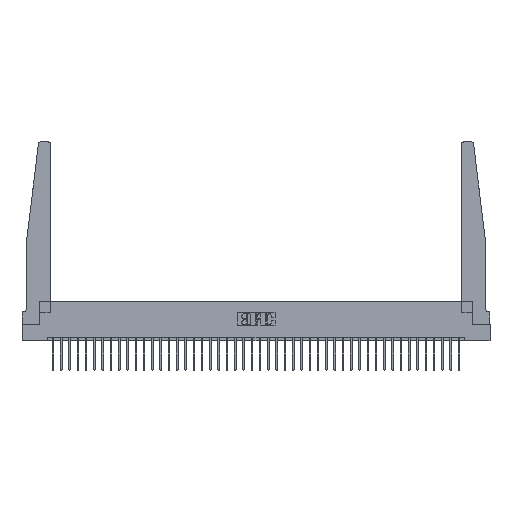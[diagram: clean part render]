
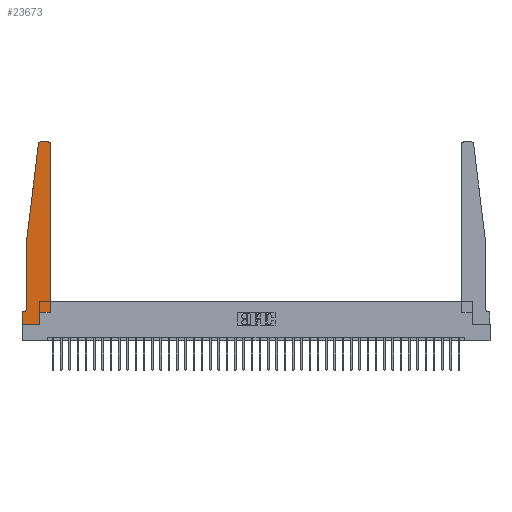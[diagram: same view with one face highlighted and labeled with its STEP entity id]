
A CAD part, top view. The second image highlights one B-rep face of the part: STEP entity #23673.
In plain terms, the highlighted planar face has unit normal (0, 0, 1).
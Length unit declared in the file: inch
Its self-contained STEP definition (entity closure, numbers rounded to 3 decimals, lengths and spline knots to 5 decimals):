
#261 = EDGE_LOOP ( 'NONE', ( #20684, #26477, #16631, #6091, #30524, #27600, #25866, #5834, #3191, #8412, #11395, #14892 ) ) ;
#293 = CARTESIAN_POINT ( 'NONE',  ( 0., 0.1875, 0.37 ) ) ;
#601 = DIRECTION ( 'NONE',  ( 1., 0., 0. ) ) ;
#1388 = CARTESIAN_POINT ( 'NONE',  ( 0.065, 1.25, 0.37 ) ) ;
#1584 = AXIS2_PLACEMENT_3D ( 'NONE', #11015, #36303, #19502 ) ;
#1932 = CARTESIAN_POINT ( 'NONE',  ( 0.395, 2.75, 0.37 ) ) ;
#2419 = EDGE_CURVE ( 'NONE', #19252, #33587, #9797, .T. ) ;
#3022 = VERTEX_POINT ( 'NONE', #9951 ) ;
#3074 = VERTEX_POINT ( 'NONE', #13169 ) ;
#3191 = ORIENTED_EDGE ( 'NONE', *, *, #34899, .T. ) ;
#4273 = EDGE_CURVE ( 'NONE', #20313, #17074, #19392, .T. ) ;
#4833 = DIRECTION ( 'NONE',  ( -1., 0., 0. ) ) ;
#5473 = CARTESIAN_POINT ( 'NONE',  ( 0.015, 0.1875, 0.37 ) ) ;
#5834 = ORIENTED_EDGE ( 'NONE', *, *, #20996, .T. ) ;
#6091 = ORIENTED_EDGE ( 'NONE', *, *, #18417, .T. ) ;
#6622 = VECTOR ( 'NONE', #32707, 39.37008 ) ;
#6654 = DIRECTION ( 'NONE',  ( 0., 1., 0. ) ) ;
#6758 = EDGE_CURVE ( 'NONE', #3022, #12682, #29801, .T. ) ;
#8298 = AXIS2_PLACEMENT_3D ( 'NONE', #293, #34190, #30541 ) ;
#8412 = ORIENTED_EDGE ( 'NONE', *, *, #4273, .T. ) ;
#8420 = LINE ( 'NONE', #16479, #15022 ) ;
#8634 = VERTEX_POINT ( 'NONE', #17667 ) ;
#8946 = EDGE_CURVE ( 'NONE', #20688, #19252, #32257, .T. ) ;
#9797 = CIRCLE ( 'NONE', #1584, 0.03 ) ;
#9951 = CARTESIAN_POINT ( 'NONE',  ( 0., 0.1875, 0.37 ) ) ;
#11015 = CARTESIAN_POINT ( 'NONE',  ( 0.27653, 2.72, 0.37 ) ) ;
#11395 = ORIENTED_EDGE ( 'NONE', *, *, #22938, .T. ) ;
#12236 = CARTESIAN_POINT ( 'NONE',  ( 0.2605, 0.18, 0.37 ) ) ;
#12353 = CARTESIAN_POINT ( 'NONE',  ( 0.27653, 2.75, 0.37 ) ) ;
#12682 = VERTEX_POINT ( 'NONE', #31662 ) ;
#13169 = CARTESIAN_POINT ( 'NONE',  ( 0.065, 1.25, 0.37 ) ) ;
#14366 = CARTESIAN_POINT ( 'NONE',  ( 0., 0., 0.37 ) ) ;
#14892 = ORIENTED_EDGE ( 'NONE', *, *, #35914, .T. ) ;
#15022 = VECTOR ( 'NONE', #22099, 39.37008 ) ;
#15377 = CARTESIAN_POINT ( 'NONE',  ( 0.425, 0.18, 0.37 ) ) ;
#15450 = EDGE_CURVE ( 'NONE', #31103, #17397, #20137, .T. ) ;
#15688 = CARTESIAN_POINT ( 'NONE',  ( 0.065, 0.1875, 0.37 ) ) ;
#16479 = CARTESIAN_POINT ( 'NONE',  ( 0.425, 0.18, 0.37 ) ) ;
#16631 = ORIENTED_EDGE ( 'NONE', *, *, #23407, .T. ) ;
#17039 = CIRCLE ( 'NONE', #25941, 0.03 ) ;
#17074 = VERTEX_POINT ( 'NONE', #15377 ) ;
#17328 = CARTESIAN_POINT ( 'NONE',  ( 0.395, 2.72, 0.37 ) ) ;
#17397 = VERTEX_POINT ( 'NONE', #5473 ) ;
#17667 = CARTESIAN_POINT ( 'NONE',  ( 0.2605, 0., 0.37 ) ) ;
#18417 = EDGE_CURVE ( 'NONE', #3074, #31103, #34608, .T. ) ;
#18793 = CARTESIAN_POINT ( 'NONE',  ( 0.425, 2.72, 0.37 ) ) ;
#18911 = CARTESIAN_POINT ( 'NONE',  ( 0.425, 0.18, 0.37 ) ) ;
#19244 = PLANE ( 'NONE',  #8298 ) ;
#19252 = VERTEX_POINT ( 'NONE', #12353 ) ;
#19392 = LINE ( 'NONE', #18911, #30805 ) ;
#19502 = DIRECTION ( 'NONE',  ( 1., 0., 0. ) ) ;
#19924 = CARTESIAN_POINT ( 'NONE',  ( 0.24675, 2.72367, 0.37 ) ) ;
#19927 = CARTESIAN_POINT ( 'NONE',  ( 0.2605, 0.18, 0.37 ) ) ;
#20000 = DIRECTION ( 'NONE',  ( 1., 0., 0. ) ) ;
#20137 = CIRCLE ( 'NONE', #31243, 0.05 ) ;
#20313 = VERTEX_POINT ( 'NONE', #19927 ) ;
#20684 = ORIENTED_EDGE ( 'NONE', *, *, #8946, .T. ) ;
#20688 = VERTEX_POINT ( 'NONE', #1932 ) ;
#20996 = EDGE_CURVE ( 'NONE', #12682, #8634, #30130, .T. ) ;
#21135 = VECTOR ( 'NONE', #26682, 39.37008 ) ;
#21703 = DIRECTION ( 'NONE',  ( 0., 0., -1. ) ) ;
#22027 = LINE ( 'NONE', #1388, #21135 ) ;
#22099 = DIRECTION ( 'NONE',  ( 0., 1., 0. ) ) ;
#22491 = LINE ( 'NONE', #15688, #6622 ) ;
#22868 = FACE_OUTER_BOUND ( 'NONE', #261, .T. ) ;
#22938 = EDGE_CURVE ( 'NONE', #17074, #33707, #8420, .T. ) ;
#23176 = VECTOR ( 'NONE', #24144, 39.37008 ) ;
#23407 = EDGE_CURVE ( 'NONE', #33587, #3074, #22027, .T. ) ;
#23673 = ADVANCED_FACE ( 'NONE', ( #22868 ), #19244, .T. ) ;
#24144 = DIRECTION ( 'NONE',  ( 0., -1., 0. ) ) ;
#24748 = CARTESIAN_POINT ( 'NONE',  ( 0.015, 0.2375, 0.37 ) ) ;
#25866 = ORIENTED_EDGE ( 'NONE', *, *, #6758, .T. ) ;
#25941 = AXIS2_PLACEMENT_3D ( 'NONE', #17328, #31327, #601 ) ;
#26477 = ORIENTED_EDGE ( 'NONE', *, *, #2419, .T. ) ;
#26682 = DIRECTION ( 'NONE',  ( -0.122, -0.992, 0. ) ) ;
#27334 = EDGE_CURVE ( 'NONE', #17397, #3022, #22491, .T. ) ;
#27590 = DIRECTION ( 'NONE',  ( 0., -1., 0. ) ) ;
#27600 = ORIENTED_EDGE ( 'NONE', *, *, #27334, .T. ) ;
#29801 = LINE ( 'NONE', #30075, #23176 ) ;
#30075 = CARTESIAN_POINT ( 'NONE',  ( 0., 0., 0.37 ) ) ;
#30103 = VECTOR ( 'NONE', #34036, 39.37008 ) ;
#30130 = LINE ( 'NONE', #14366, #31866 ) ;
#30524 = ORIENTED_EDGE ( 'NONE', *, *, #15450, .T. ) ;
#30541 = DIRECTION ( 'NONE',  ( 1., 0., 0. ) ) ;
#30805 = VECTOR ( 'NONE', #36088, 39.37008 ) ;
#31103 = VERTEX_POINT ( 'NONE', #34172 ) ;
#31185 = VECTOR ( 'NONE', #6654, 39.37008 ) ;
#31243 = AXIS2_PLACEMENT_3D ( 'NONE', #24748, #21703, #4833 ) ;
#31327 = DIRECTION ( 'NONE',  ( 0., 0., 1. ) ) ;
#31662 = CARTESIAN_POINT ( 'NONE',  ( 0., 0., 0.37 ) ) ;
#31866 = VECTOR ( 'NONE', #20000, 39.37008 ) ;
#32257 = LINE ( 'NONE', #33642, #30103 ) ;
#32464 = LINE ( 'NONE', #12236, #31185 ) ;
#32632 = CARTESIAN_POINT ( 'NONE',  ( 0.065, 1.25, 0.37 ) ) ;
#32707 = DIRECTION ( 'NONE',  ( -1., 0., 0. ) ) ;
#33587 = VERTEX_POINT ( 'NONE', #19924 ) ;
#33642 = CARTESIAN_POINT ( 'NONE',  ( 0.25, 2.75, 0.37 ) ) ;
#33707 = VERTEX_POINT ( 'NONE', #18793 ) ;
#34036 = DIRECTION ( 'NONE',  ( -1., 0., 0. ) ) ;
#34172 = CARTESIAN_POINT ( 'NONE',  ( 0.065, 0.2375, 0.37 ) ) ;
#34190 = DIRECTION ( 'NONE',  ( 0., 0., 1. ) ) ;
#34608 = LINE ( 'NONE', #32632, #35959 ) ;
#34899 = EDGE_CURVE ( 'NONE', #8634, #20313, #32464, .T. ) ;
#35914 = EDGE_CURVE ( 'NONE', #33707, #20688, #17039, .T. ) ;
#35959 = VECTOR ( 'NONE', #27590, 39.37008 ) ;
#36088 = DIRECTION ( 'NONE',  ( 1., 0., 0. ) ) ;
#36303 = DIRECTION ( 'NONE',  ( 0., 0., 1. ) ) ;
